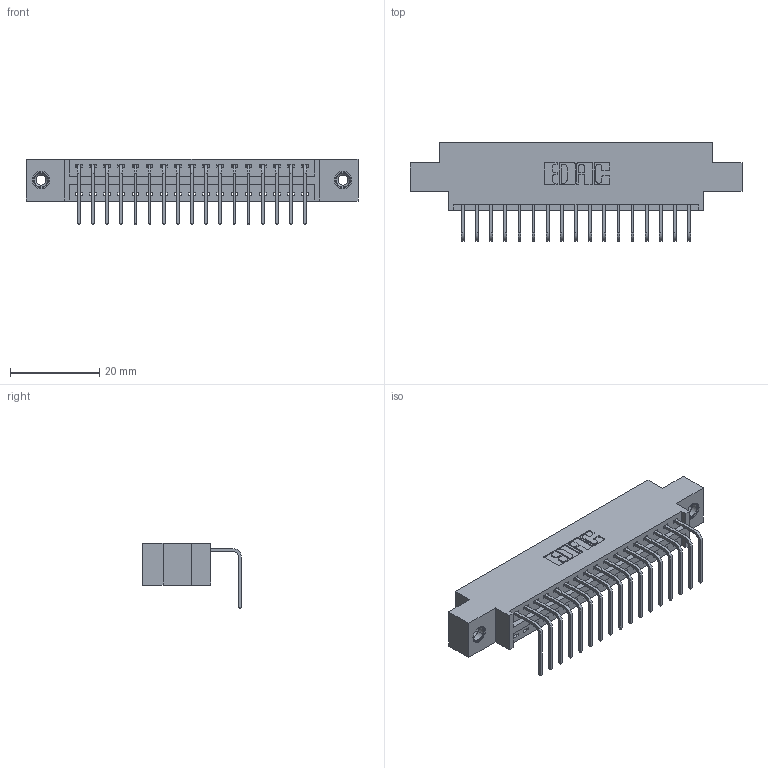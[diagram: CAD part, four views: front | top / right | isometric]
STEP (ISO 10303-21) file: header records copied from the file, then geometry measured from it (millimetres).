
FILE_DESCRIPTION (( 'STEP AP203' ), '1' );
FILE_NAME ('396-017-558-608.STEP', '2019-11-01T05:57:31', ( '' ), ( '' ), 'SwSTEP 2.0', 'SolidWorks 2016', '' );
FILE_SCHEMA (( 'CONFIG_CONTROL_DESIGN' ));
Length unit declared in the file: inch
Products named in the file (4): 396-017-558-608; 346 Part_0.170 Offset - 0.156 Dia-TI; 345-292-001_558 Tail - 2; 345-250-001_345-250-003-102
Assembly tree (20 placements, depth 2):
  396-017-558-608
    346 Part_0.170 Offset - 0.156 Dia-TI
    345-292-001_558 Tail - 2  x17
    345-250-001_345-250-003-102  x2
Bounding box: 74.55 x 22.16 x 14.73 mm (x, y, z)
Volume: 6859.3 mm3; surface area: 8823.4 mm2
Topology: 20 solids, 20 shells, 1206 faces, 3571 edges, 2350 vertices
Faces by surface type: plane 826, cylinder 364, cone 12, torus 4
Entity records: 15318 total; most frequent: CARTESIAN_POINT 2618, ORIENTED_EDGE 2562, DIRECTION 2365, EDGE_CURVE 1281, LINE 1061, VECTOR 1061, VERTEX_POINT 848, AXIS2_PLACEMENT_3D 652
